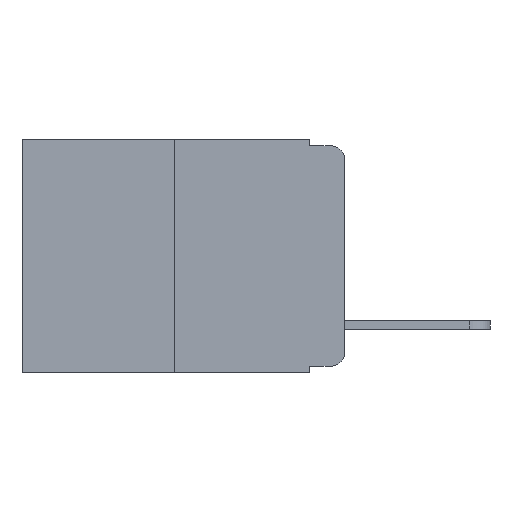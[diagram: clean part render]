
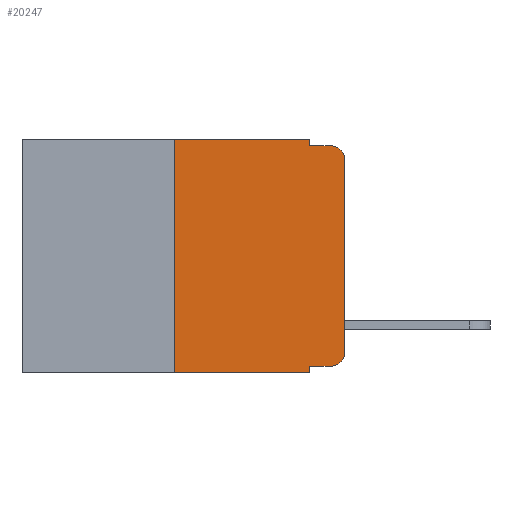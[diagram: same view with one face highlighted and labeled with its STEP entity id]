
A CAD part, left-side view. The second image highlights one B-rep face of the part: STEP entity #20247.
In plain terms, the highlighted planar face has unit normal (-1, 0, 0).
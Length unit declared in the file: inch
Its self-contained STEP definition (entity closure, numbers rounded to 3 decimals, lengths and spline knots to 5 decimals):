
#174 = VECTOR ( 'NONE', #25336, 39.37008 ) ;
#2532 = CARTESIAN_POINT ( 'NONE',  ( 0., 0.051, -0.333 ) ) ;
#3480 = CARTESIAN_POINT ( 'NONE',  ( 0., 0.051, -0.01 ) ) ;
#3513 = DIRECTION ( 'NONE',  ( 0., -1., 0. ) ) ;
#3665 = LINE ( 'NONE', #18062, #14631 ) ;
#4007 = DIRECTION ( 'NONE',  ( 1., 0., 0. ) ) ;
#4188 = VECTOR ( 'NONE', #8554, 39.37008 ) ;
#4573 = CARTESIAN_POINT ( 'NONE',  ( 0., 0., 0. ) ) ;
#4706 = EDGE_CURVE ( 'NONE', #4800, #9845, #16632, .T. ) ;
#4800 = VERTEX_POINT ( 'NONE', #16783 ) ;
#4898 = CARTESIAN_POINT ( 'NONE',  ( 0., 0.051, 0. ) ) ;
#5002 = VERTEX_POINT ( 'NONE', #25873 ) ;
#5015 = LINE ( 'NONE', #3480, #21715 ) ;
#5115 = LINE ( 'NONE', #4573, #9828 ) ;
#5682 = EDGE_CURVE ( 'NONE', #11948, #23213, #23075, .T. ) ;
#6270 = VECTOR ( 'NONE', #22609, 39.37008 ) ;
#6367 = ORIENTED_EDGE ( 'NONE', *, *, #23787, .T. ) ;
#6432 = ORIENTED_EDGE ( 'NONE', *, *, #6691, .T. ) ;
#6691 = EDGE_CURVE ( 'NONE', #13902, #5002, #12946, .T. ) ;
#6897 = AXIS2_PLACEMENT_3D ( 'NONE', #11073, #11023, #11016 ) ;
#7097 = EDGE_CURVE ( 'NONE', #10966, #5002, #5015, .T. ) ;
#7099 = ORIENTED_EDGE ( 'NONE', *, *, #7097, .F. ) ;
#7148 = ORIENTED_EDGE ( 'NONE', *, *, #8187, .F. ) ;
#7208 = ORIENTED_EDGE ( 'NONE', *, *, #5682, .F. ) ;
#7469 = ORIENTED_EDGE ( 'NONE', *, *, #9201, .F. ) ;
#7624 = ORIENTED_EDGE ( 'NONE', *, *, #4706, .T. ) ;
#8003 = CARTESIAN_POINT ( 'NONE',  ( 0., 0.051, -0.01 ) ) ;
#8107 = ORIENTED_EDGE ( 'NONE', *, *, #9784, .F. ) ;
#8187 = EDGE_CURVE ( 'NONE', #23213, #10966, #10297, .T. ) ;
#8486 = ORIENTED_EDGE ( 'NONE', *, *, #10782, .T. ) ;
#8554 = DIRECTION ( 'NONE',  ( 0., 0., -1. ) ) ;
#8644 = ORIENTED_EDGE ( 'NONE', *, *, #12689, .T. ) ;
#8775 = CARTESIAN_POINT ( 'NONE',  ( 0., 0.051, 0. ) ) ;
#9201 = EDGE_CURVE ( 'NONE', #4800, #11948, #17517, .T. ) ;
#9235 = FACE_OUTER_BOUND ( 'NONE', #17069, .T. ) ;
#9784 = EDGE_CURVE ( 'NONE', #12519, #9845, #23931, .T. ) ;
#9828 = VECTOR ( 'NONE', #24954, 39.37008 ) ;
#9845 = VERTEX_POINT ( 'NONE', #11540 ) ;
#10297 = LINE ( 'NONE', #8775, #4188 ) ;
#10674 = PLANE ( 'NONE',  #23779 ) ;
#10762 = CARTESIAN_POINT ( 'NONE',  ( 0., 0.473, 0. ) ) ;
#10782 = EDGE_CURVE ( 'NONE', #12519, #18260, #3665, .T. ) ;
#10966 = VERTEX_POINT ( 'NONE', #8003 ) ;
#11016 = DIRECTION ( 'NONE',  ( 0., 0., -1. ) ) ;
#11023 = DIRECTION ( 'NONE',  ( -1., 0., 0. ) ) ;
#11073 = CARTESIAN_POINT ( 'NONE',  ( 0., 0.02, -0.03 ) ) ;
#11540 = CARTESIAN_POINT ( 'NONE',  ( 0., 0.051, -0.343 ) ) ;
#11948 = VERTEX_POINT ( 'NONE', #12446 ) ;
#12446 = CARTESIAN_POINT ( 'NONE',  ( 0., 0.25, 0. ) ) ;
#12519 = VERTEX_POINT ( 'NONE', #2532 ) ;
#12657 = CARTESIAN_POINT ( 'NONE',  ( 0., 0.051, 0. ) ) ;
#12689 = EDGE_CURVE ( 'NONE', #18260, #26449, #18855, .T. ) ;
#12946 = CIRCLE ( 'NONE', #6897, 0.02 ) ;
#13047 = DIRECTION ( 'NONE',  ( 0., 0., -1. ) ) ;
#13902 = VERTEX_POINT ( 'NONE', #14171 ) ;
#14171 = CARTESIAN_POINT ( 'NONE',  ( 0., 0., -0.03 ) ) ;
#14631 = VECTOR ( 'NONE', #18184, 39.37008 ) ;
#15661 = AXIS2_PLACEMENT_3D ( 'NONE', #25960, #25867, #25863 ) ;
#16632 = LINE ( 'NONE', #23271, #26125 ) ;
#16783 = CARTESIAN_POINT ( 'NONE',  ( 0., 0.25, -0.343 ) ) ;
#17069 = EDGE_LOOP ( 'NONE', ( #6367, #6432, #7099, #7148, #7208, #7469, #7624, #8107, #8486, #8644 ) ) ;
#17366 = CARTESIAN_POINT ( 'NONE',  ( 0., 0., -0.313 ) ) ;
#17517 = LINE ( 'NONE', #22801, #6270 ) ;
#18062 = CARTESIAN_POINT ( 'NONE',  ( 0., 0.051, -0.333 ) ) ;
#18184 = DIRECTION ( 'NONE',  ( 0., -1., 0. ) ) ;
#18260 = VERTEX_POINT ( 'NONE', #22935 ) ;
#18794 = VECTOR ( 'NONE', #13047, 39.37008 ) ;
#18855 = CIRCLE ( 'NONE', #15661, 0.02 ) ;
#18934 = DIRECTION ( 'NONE',  ( 0., 0., -1. ) ) ;
#20247 = ADVANCED_FACE ( 'NONE', ( #9235 ), #10674, .F. ) ;
#21715 = VECTOR ( 'NONE', #3513, 39.37008 ) ;
#22609 = DIRECTION ( 'NONE',  ( 0., 0., 1. ) ) ;
#22801 = CARTESIAN_POINT ( 'NONE',  ( 0., 0.25, 0. ) ) ;
#22935 = CARTESIAN_POINT ( 'NONE',  ( 0., 0.02, -0.333 ) ) ;
#23075 = LINE ( 'NONE', #25237, #174 ) ;
#23213 = VERTEX_POINT ( 'NONE', #4898 ) ;
#23271 = CARTESIAN_POINT ( 'NONE',  ( 0., 0.473, -0.343 ) ) ;
#23656 = DIRECTION ( 'NONE',  ( 0., -1., 0. ) ) ;
#23779 = AXIS2_PLACEMENT_3D ( 'NONE', #10762, #4007, #18934 ) ;
#23787 = EDGE_CURVE ( 'NONE', #26449, #13902, #5115, .T. ) ;
#23931 = LINE ( 'NONE', #12657, #18794 ) ;
#24954 = DIRECTION ( 'NONE',  ( 0., 0., 1. ) ) ;
#25237 = CARTESIAN_POINT ( 'NONE',  ( 0., 0.473, 0. ) ) ;
#25336 = DIRECTION ( 'NONE',  ( 0., -1., 0. ) ) ;
#25863 = DIRECTION ( 'NONE',  ( 0., 0., -1. ) ) ;
#25867 = DIRECTION ( 'NONE',  ( -1., 0., 0. ) ) ;
#25873 = CARTESIAN_POINT ( 'NONE',  ( 0., 0.02, -0.01 ) ) ;
#25960 = CARTESIAN_POINT ( 'NONE',  ( 0., 0.02, -0.313 ) ) ;
#26125 = VECTOR ( 'NONE', #23656, 39.37008 ) ;
#26449 = VERTEX_POINT ( 'NONE', #17366 ) ;
